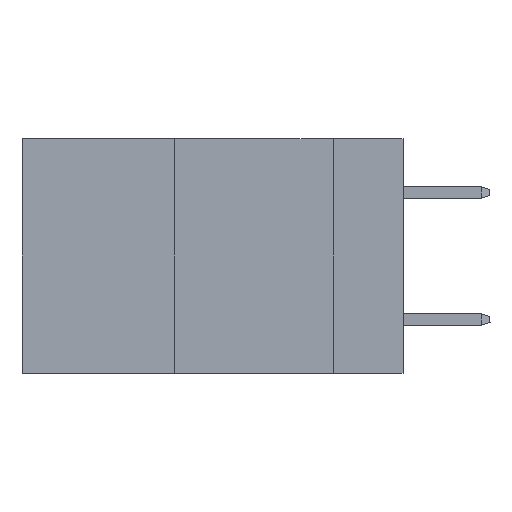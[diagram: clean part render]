
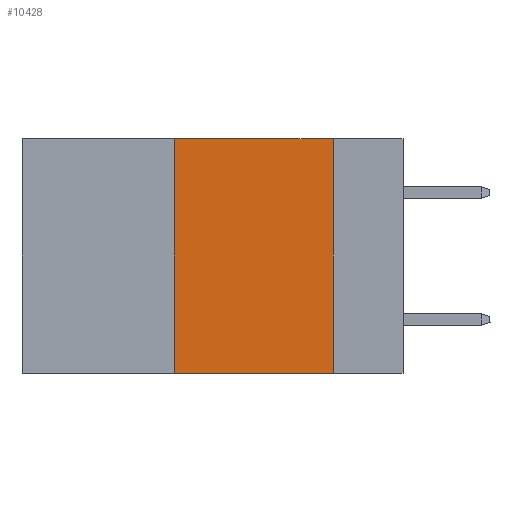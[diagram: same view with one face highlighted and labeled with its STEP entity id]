
A CAD part, left-side view. The second image highlights one B-rep face of the part: STEP entity #10428.
In plain terms, the highlighted planar face has unit normal (-1, 0, 0).
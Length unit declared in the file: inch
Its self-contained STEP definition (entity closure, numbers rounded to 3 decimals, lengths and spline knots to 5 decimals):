
#71 = AXIS2_PLACEMENT_3D ( 'NONE', #11080, #16527, #2018 ) ;
#209 = VERTEX_POINT ( 'NONE', #11846 ) ;
#230 = FACE_OUTER_BOUND ( 'NONE', #602, .T. ) ;
#602 = EDGE_LOOP ( 'NONE', ( #20216, #2806, #14650, #12437 ) ) ;
#1167 = LINE ( 'NONE', #15450, #9388 ) ;
#1174 = VECTOR ( 'NONE', #15809, 39.37008 ) ;
#2018 = DIRECTION ( 'NONE',  ( 0., 0., -1. ) ) ;
#2806 = ORIENTED_EDGE ( 'NONE', *, *, #19404, .F. ) ;
#3182 = LINE ( 'NONE', #8933, #16305 ) ;
#3689 = VECTOR ( 'NONE', #21154, 39.37008 ) ;
#4325 = VERTEX_POINT ( 'NONE', #12471 ) ;
#5468 = EDGE_CURVE ( 'NONE', #19856, #209, #13895, .T. ) ;
#8650 = LINE ( 'NONE', #23044, #3689 ) ;
#8933 = CARTESIAN_POINT ( 'NONE',  ( 0., 0.6, 0. ) ) ;
#9388 = VECTOR ( 'NONE', #22628, 39.37008 ) ;
#10428 = ADVANCED_FACE ( 'NONE', ( #230 ), #18182, .F. ) ;
#11080 = CARTESIAN_POINT ( 'NONE',  ( 0., 0.6, 0. ) ) ;
#11846 = CARTESIAN_POINT ( 'NONE',  ( 0., 0.36, 0. ) ) ;
#12437 = ORIENTED_EDGE ( 'NONE', *, *, #17144, .T. ) ;
#12471 = CARTESIAN_POINT ( 'NONE',  ( 0., 0.11, 0. ) ) ;
#12494 = EDGE_CURVE ( 'NONE', #4325, #12685, #1167, .T. ) ;
#12685 = VERTEX_POINT ( 'NONE', #18265 ) ;
#13895 = LINE ( 'NONE', #20871, #1174 ) ;
#14650 = ORIENTED_EDGE ( 'NONE', *, *, #5468, .F. ) ;
#15450 = CARTESIAN_POINT ( 'NONE',  ( 0., 0.11, 0. ) ) ;
#15809 = DIRECTION ( 'NONE',  ( 0., 0., 1. ) ) ;
#16305 = VECTOR ( 'NONE', #22994, 39.37008 ) ;
#16527 = DIRECTION ( 'NONE',  ( 1., 0., 0. ) ) ;
#17144 = EDGE_CURVE ( 'NONE', #19856, #12685, #8650, .T. ) ;
#18182 = PLANE ( 'NONE',  #71 ) ;
#18265 = CARTESIAN_POINT ( 'NONE',  ( 0., 0.11, -0.37 ) ) ;
#19404 = EDGE_CURVE ( 'NONE', #209, #4325, #3182, .T. ) ;
#19856 = VERTEX_POINT ( 'NONE', #22850 ) ;
#20216 = ORIENTED_EDGE ( 'NONE', *, *, #12494, .F. ) ;
#20871 = CARTESIAN_POINT ( 'NONE',  ( 0., 0.36, 0. ) ) ;
#21154 = DIRECTION ( 'NONE',  ( 0., -1., 0. ) ) ;
#22628 = DIRECTION ( 'NONE',  ( 0., 0., -1. ) ) ;
#22850 = CARTESIAN_POINT ( 'NONE',  ( 0., 0.36, -0.37 ) ) ;
#22994 = DIRECTION ( 'NONE',  ( 0., -1., 0. ) ) ;
#23044 = CARTESIAN_POINT ( 'NONE',  ( 0., 0.6, -0.37 ) ) ;
